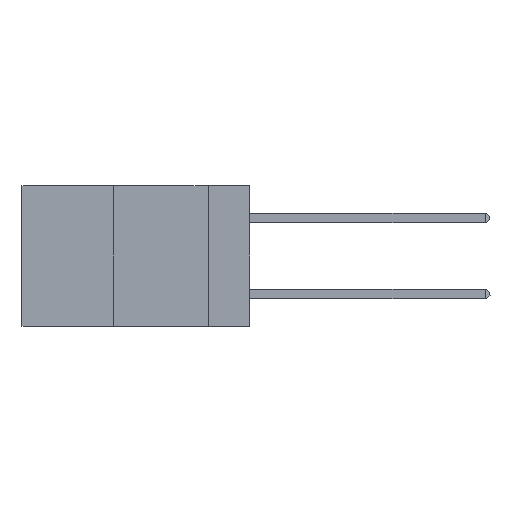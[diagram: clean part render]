
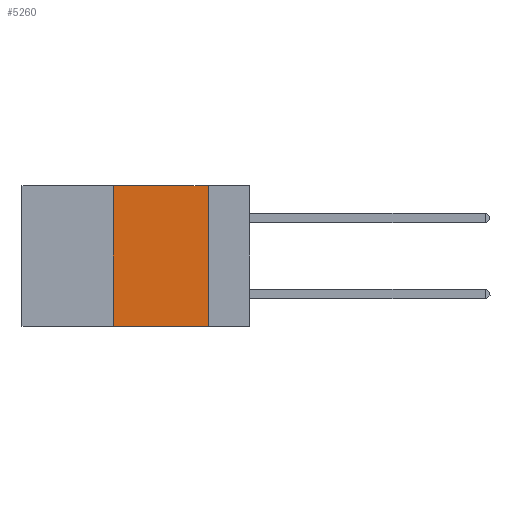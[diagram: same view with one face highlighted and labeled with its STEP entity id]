
A CAD part, left-side view. The second image highlights one B-rep face of the part: STEP entity #5260.
In plain terms, the highlighted planar face has unit normal (-1, 0, 0).
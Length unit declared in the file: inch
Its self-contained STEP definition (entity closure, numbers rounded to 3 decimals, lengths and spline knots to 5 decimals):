
#528 = FACE_OUTER_BOUND ( 'NONE', #9349, .T. ) ;
#1324 = CARTESIAN_POINT ( 'NONE',  ( 0., 0.36, 0. ) ) ;
#1376 = DIRECTION ( 'NONE',  ( 0., 0., 1. ) ) ;
#1405 = VECTOR ( 'NONE', #7337, 39.37008 ) ;
#2216 = VECTOR ( 'NONE', #5192, 39.37008 ) ;
#2624 = CARTESIAN_POINT ( 'NONE',  ( 0., 0.11, 0. ) ) ;
#3706 = AXIS2_PLACEMENT_3D ( 'NONE', #6357, #9384, #7392 ) ;
#3872 = VECTOR ( 'NONE', #7128, 39.37008 ) ;
#4671 = LINE ( 'NONE', #9416, #1405 ) ;
#4836 = LINE ( 'NONE', #9108, #3872 ) ;
#4988 = ORIENTED_EDGE ( 'NONE', *, *, #9924, .T. ) ;
#5192 = DIRECTION ( 'NONE',  ( 0., 0., -1. ) ) ;
#5249 = LINE ( 'NONE', #1324, #6954 ) ;
#5260 = ADVANCED_FACE ( 'NONE', ( #528 ), #10307, .F. ) ;
#5269 = CARTESIAN_POINT ( 'NONE',  ( 0., 0.11, 0. ) ) ;
#5522 = CARTESIAN_POINT ( 'NONE',  ( 0., 0.36, -0.37 ) ) ;
#5621 = VERTEX_POINT ( 'NONE', #2624 ) ;
#6357 = CARTESIAN_POINT ( 'NONE',  ( 0., 0.6, 0. ) ) ;
#6521 = EDGE_CURVE ( 'NONE', #7723, #5621, #4836, .T. ) ;
#6549 = EDGE_CURVE ( 'NONE', #5621, #10913, #11515, .T. ) ;
#6954 = VECTOR ( 'NONE', #1376, 39.37008 ) ;
#7123 = ORIENTED_EDGE ( 'NONE', *, *, #6549, .F. ) ;
#7128 = DIRECTION ( 'NONE',  ( 0., -1., 0. ) ) ;
#7337 = DIRECTION ( 'NONE',  ( 0., -1., 0. ) ) ;
#7392 = DIRECTION ( 'NONE',  ( 0., 0., -1. ) ) ;
#7723 = VERTEX_POINT ( 'NONE', #10039 ) ;
#8902 = CARTESIAN_POINT ( 'NONE',  ( 0., 0.11, -0.37 ) ) ;
#9053 = ORIENTED_EDGE ( 'NONE', *, *, #6521, .F. ) ;
#9108 = CARTESIAN_POINT ( 'NONE',  ( 0., 0.6, 0. ) ) ;
#9349 = EDGE_LOOP ( 'NONE', ( #7123, #9053, #9598, #4988 ) ) ;
#9384 = DIRECTION ( 'NONE',  ( 1., 0., 0. ) ) ;
#9416 = CARTESIAN_POINT ( 'NONE',  ( 0., 0.6, -0.37 ) ) ;
#9475 = VERTEX_POINT ( 'NONE', #5522 ) ;
#9598 = ORIENTED_EDGE ( 'NONE', *, *, #12579, .F. ) ;
#9924 = EDGE_CURVE ( 'NONE', #9475, #10913, #4671, .T. ) ;
#10039 = CARTESIAN_POINT ( 'NONE',  ( 0., 0.36, 0. ) ) ;
#10307 = PLANE ( 'NONE',  #3706 ) ;
#10913 = VERTEX_POINT ( 'NONE', #8902 ) ;
#11515 = LINE ( 'NONE', #5269, #2216 ) ;
#12579 = EDGE_CURVE ( 'NONE', #9475, #7723, #5249, .T. ) ;
